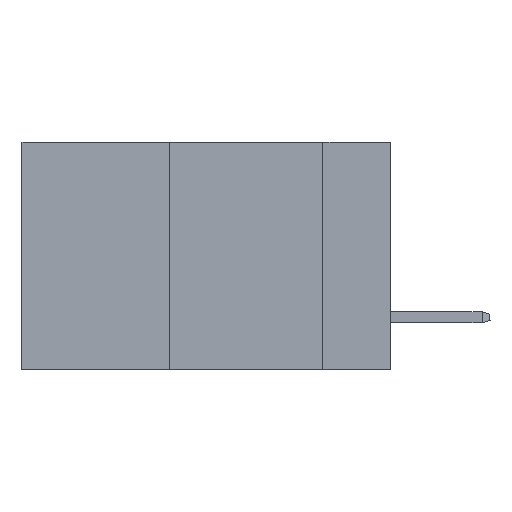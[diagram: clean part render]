
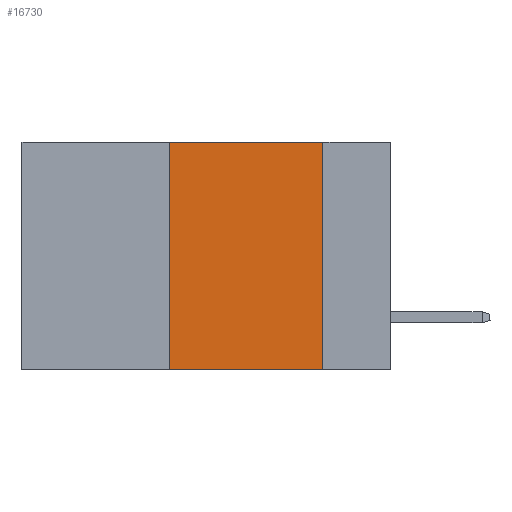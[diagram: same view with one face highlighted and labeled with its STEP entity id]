
A CAD part, left-side view. The second image highlights one B-rep face of the part: STEP entity #16730.
In plain terms, the highlighted planar face has unit normal (-1, 0, 0).
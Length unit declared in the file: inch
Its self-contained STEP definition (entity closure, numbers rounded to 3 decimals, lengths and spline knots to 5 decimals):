
#51 = CARTESIAN_POINT ( 'NONE',  ( 0., 0.36, 0. ) ) ;
#418 = DIRECTION ( 'NONE',  ( 0., -1., 0. ) ) ;
#1272 = CARTESIAN_POINT ( 'NONE',  ( 0., 0.11, -0.37 ) ) ;
#1566 = DIRECTION ( 'NONE',  ( 0., 0., -1. ) ) ;
#1719 = VERTEX_POINT ( 'NONE', #1272 ) ;
#1975 = VERTEX_POINT ( 'NONE', #14303 ) ;
#2772 = CARTESIAN_POINT ( 'NONE',  ( 0., 0.11, 0. ) ) ;
#2912 = CARTESIAN_POINT ( 'NONE',  ( 0., 0.6, 0. ) ) ;
#4238 = VECTOR ( 'NONE', #6153, 39.37008 ) ;
#4398 = ORIENTED_EDGE ( 'NONE', *, *, #12583, .T. ) ;
#4994 = LINE ( 'NONE', #2912, #13196 ) ;
#5143 = ORIENTED_EDGE ( 'NONE', *, *, #14081, .F. ) ;
#5426 = LINE ( 'NONE', #51, #11552 ) ;
#5512 = ORIENTED_EDGE ( 'NONE', *, *, #10595, .F. ) ;
#5606 = CARTESIAN_POINT ( 'NONE',  ( 0., 0.6, 0. ) ) ;
#6128 = CARTESIAN_POINT ( 'NONE',  ( 0., 0.11, 0. ) ) ;
#6153 = DIRECTION ( 'NONE',  ( 0., -1., 0. ) ) ;
#7400 = FACE_OUTER_BOUND ( 'NONE', #16957, .T. ) ;
#7657 = AXIS2_PLACEMENT_3D ( 'NONE', #5606, #8144, #1566 ) ;
#7705 = CARTESIAN_POINT ( 'NONE',  ( 0., 0.6, -0.37 ) ) ;
#7776 = VERTEX_POINT ( 'NONE', #15156 ) ;
#8144 = DIRECTION ( 'NONE',  ( 1., 0., 0. ) ) ;
#8361 = LINE ( 'NONE', #7705, #4238 ) ;
#8521 = EDGE_CURVE ( 'NONE', #1975, #7776, #5426, .T. ) ;
#9463 = PLANE ( 'NONE',  #7657 ) ;
#10369 = ORIENTED_EDGE ( 'NONE', *, *, #8521, .F. ) ;
#10595 = EDGE_CURVE ( 'NONE', #15594, #1719, #11716, .T. ) ;
#11552 = VECTOR ( 'NONE', #13228, 39.37008 ) ;
#11716 = LINE ( 'NONE', #2772, #16012 ) ;
#12583 = EDGE_CURVE ( 'NONE', #1975, #1719, #8361, .T. ) ;
#13114 = DIRECTION ( 'NONE',  ( 0., 0., -1. ) ) ;
#13196 = VECTOR ( 'NONE', #418, 39.37008 ) ;
#13228 = DIRECTION ( 'NONE',  ( 0., 0., 1. ) ) ;
#14081 = EDGE_CURVE ( 'NONE', #7776, #15594, #4994, .T. ) ;
#14303 = CARTESIAN_POINT ( 'NONE',  ( 0., 0.36, -0.37 ) ) ;
#15156 = CARTESIAN_POINT ( 'NONE',  ( 0., 0.36, 0. ) ) ;
#15594 = VERTEX_POINT ( 'NONE', #6128 ) ;
#16012 = VECTOR ( 'NONE', #13114, 39.37008 ) ;
#16730 = ADVANCED_FACE ( 'NONE', ( #7400 ), #9463, .F. ) ;
#16957 = EDGE_LOOP ( 'NONE', ( #5512, #5143, #10369, #4398 ) ) ;
